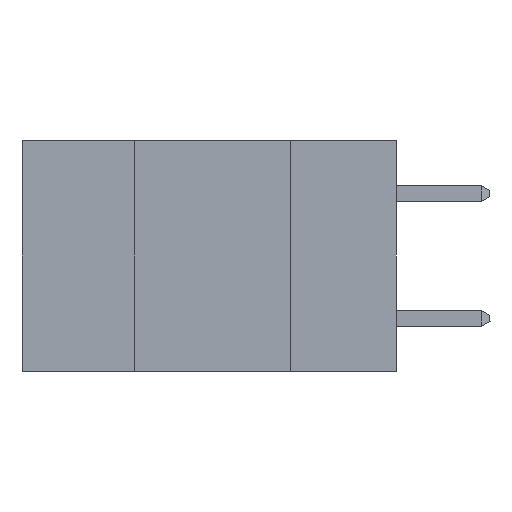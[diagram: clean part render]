
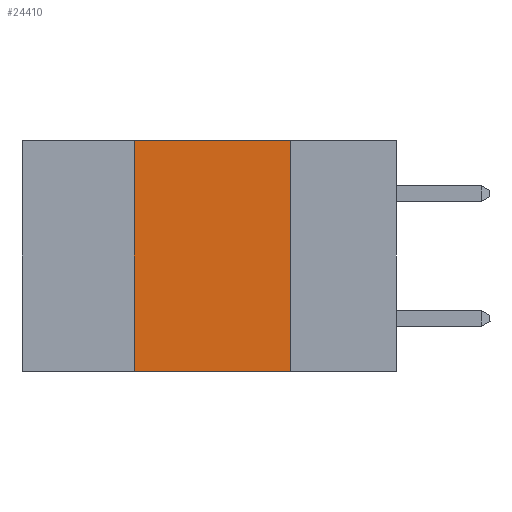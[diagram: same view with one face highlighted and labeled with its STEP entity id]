
A CAD part, left-side view. The second image highlights one B-rep face of the part: STEP entity #24410.
In plain terms, the highlighted planar face has unit normal (-1, 0, 0).
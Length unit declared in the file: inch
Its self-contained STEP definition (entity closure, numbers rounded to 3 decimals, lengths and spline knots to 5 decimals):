
#320 = LINE ( 'NONE', #3768, #22221 ) ;
#1888 = CARTESIAN_POINT ( 'NONE',  ( 0., 0.6, 0. ) ) ;
#2367 = EDGE_CURVE ( 'NONE', #26372, #19710, #20938, .T. ) ;
#3768 = CARTESIAN_POINT ( 'NONE',  ( 0., 0.17, -0.37 ) ) ;
#4034 = DIRECTION ( 'NONE',  ( 0., 0., -1. ) ) ;
#5525 = DIRECTION ( 'NONE',  ( 0., -1., 0. ) ) ;
#5764 = CARTESIAN_POINT ( 'NONE',  ( 0., 0.17, 0. ) ) ;
#6428 = CARTESIAN_POINT ( 'NONE',  ( 0., 0.6, 0. ) ) ;
#7471 = ORIENTED_EDGE ( 'NONE', *, *, #27232, .F. ) ;
#8340 = CARTESIAN_POINT ( 'NONE',  ( 0., 0.42, 0. ) ) ;
#9534 = EDGE_LOOP ( 'NONE', ( #7471, #19300, #24848, #14400 ) ) ;
#11575 = VECTOR ( 'NONE', #5525, 39.37008 ) ;
#11617 = DIRECTION ( 'NONE',  ( 0., 0., 1. ) ) ;
#11645 = CARTESIAN_POINT ( 'NONE',  ( 0., 0.42, -0.37 ) ) ;
#14400 = ORIENTED_EDGE ( 'NONE', *, *, #16084, .T. ) ;
#14473 = DIRECTION ( 'NONE',  ( 0., 0., -1. ) ) ;
#14576 = CARTESIAN_POINT ( 'NONE',  ( 0., 0.42, -0.37 ) ) ;
#15369 = VECTOR ( 'NONE', #11617, 39.37008 ) ;
#15436 = AXIS2_PLACEMENT_3D ( 'NONE', #1888, #16751, #4034 ) ;
#16058 = CARTESIAN_POINT ( 'NONE',  ( 0., 0.6, -0.37 ) ) ;
#16084 = EDGE_CURVE ( 'NONE', #26372, #21404, #17134, .T. ) ;
#16751 = DIRECTION ( 'NONE',  ( 1., 0., 0. ) ) ;
#17009 = VECTOR ( 'NONE', #21049, 39.37008 ) ;
#17134 = LINE ( 'NONE', #16058, #11575 ) ;
#18352 = EDGE_CURVE ( 'NONE', #19710, #24267, #22556, .T. ) ;
#19300 = ORIENTED_EDGE ( 'NONE', *, *, #18352, .F. ) ;
#19710 = VERTEX_POINT ( 'NONE', #8340 ) ;
#19801 = CARTESIAN_POINT ( 'NONE',  ( 0., 0.17, -0.37 ) ) ;
#20876 = PLANE ( 'NONE',  #15436 ) ;
#20938 = LINE ( 'NONE', #11645, #15369 ) ;
#21049 = DIRECTION ( 'NONE',  ( 0., -1., 0. ) ) ;
#21404 = VERTEX_POINT ( 'NONE', #19801 ) ;
#22221 = VECTOR ( 'NONE', #14473, 39.37008 ) ;
#22556 = LINE ( 'NONE', #6428, #17009 ) ;
#24267 = VERTEX_POINT ( 'NONE', #5764 ) ;
#24410 = ADVANCED_FACE ( 'NONE', ( #24506 ), #20876, .F. ) ;
#24506 = FACE_OUTER_BOUND ( 'NONE', #9534, .T. ) ;
#24848 = ORIENTED_EDGE ( 'NONE', *, *, #2367, .F. ) ;
#26372 = VERTEX_POINT ( 'NONE', #14576 ) ;
#27232 = EDGE_CURVE ( 'NONE', #24267, #21404, #320, .T. ) ;
